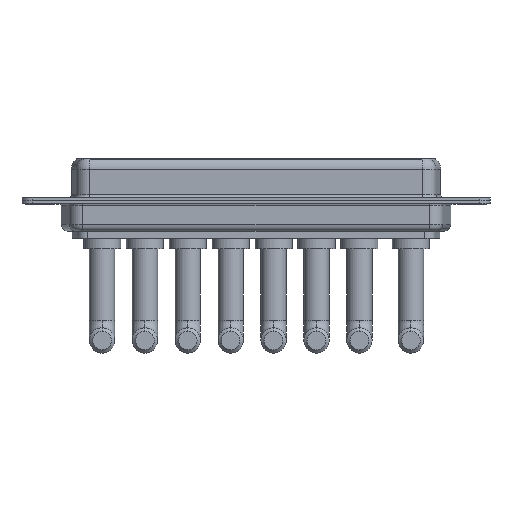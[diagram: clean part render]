
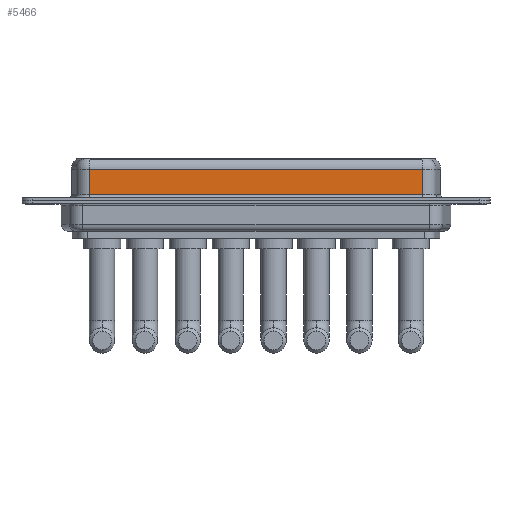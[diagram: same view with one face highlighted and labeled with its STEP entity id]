
A CAD part, front view. The second image highlights one B-rep face of the part: STEP entity #5466.
In plain terms, the highlighted planar face has unit normal (0, -1, 0).
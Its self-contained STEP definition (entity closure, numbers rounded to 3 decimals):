
#313 = ORIENTED_EDGE ( 'NONE', *, *, #11012, .F. ) ;
#325 = CARTESIAN_POINT ( 'NONE',  ( 7.038, -3.95, 0.9 ) ) ;
#837 = LINE ( 'NONE', #6211, #10198 ) ;
#909 = LINE ( 'NONE', #8097, #8647 ) ;
#1168 = EDGE_CURVE ( 'NONE', #10026, #2926, #10591, .T. ) ;
#1311 = ORIENTED_EDGE ( 'NONE', *, *, #1457, .T. ) ;
#1457 = EDGE_CURVE ( 'NONE', #5339, #10026, #9608, .T. ) ;
#2400 = CARTESIAN_POINT ( 'NONE',  ( 56.462, -3.95, 4.65 ) ) ;
#2618 = DIRECTION ( 'NONE',  ( 1., 0., 0. ) ) ;
#2660 = DIRECTION ( 'NONE',  ( 0., 0., -1. ) ) ;
#2926 = VERTEX_POINT ( 'NONE', #325 ) ;
#3051 = CARTESIAN_POINT ( 'NONE',  ( 56.462, -3.95, 6.4 ) ) ;
#3469 = ORIENTED_EDGE ( 'NONE', *, *, #6522, .T. ) ;
#4916 = DIRECTION ( 'NONE',  ( 0., 1., 0. ) ) ;
#4972 = DIRECTION ( 'NONE',  ( 0., 0., 1. ) ) ;
#5015 = CARTESIAN_POINT ( 'NONE',  ( 7.038, -3.95, 4.65 ) ) ;
#5339 = VERTEX_POINT ( 'NONE', #8720 ) ;
#5466 = ADVANCED_FACE ( 'NONE', ( #5605 ), #7546, .F. ) ;
#5553 = ORIENTED_EDGE ( 'NONE', *, *, #1168, .T. ) ;
#5587 = VECTOR ( 'NONE', #6182, 1000. ) ;
#5605 = FACE_OUTER_BOUND ( 'NONE', #8673, .T. ) ;
#5945 = CARTESIAN_POINT ( 'NONE',  ( 56.462, -3.95, 0.9 ) ) ;
#6182 = DIRECTION ( 'NONE',  ( 0., 0., -1. ) ) ;
#6211 = CARTESIAN_POINT ( 'NONE',  ( 56.462, -3.95, 6.4 ) ) ;
#6522 = EDGE_CURVE ( 'NONE', #2926, #10752, #909, .T. ) ;
#7086 = CARTESIAN_POINT ( 'NONE',  ( 7.038, -3.95, 6.4 ) ) ;
#7546 = PLANE ( 'NONE',  #10645 ) ;
#8097 = CARTESIAN_POINT ( 'NONE',  ( 56.462, -3.95, 0.9 ) ) ;
#8444 = VECTOR ( 'NONE', #11218, 1000. ) ;
#8647 = VECTOR ( 'NONE', #2618, 1000. ) ;
#8673 = EDGE_LOOP ( 'NONE', ( #313, #1311, #5553, #3469 ) ) ;
#8720 = CARTESIAN_POINT ( 'NONE',  ( 56.462, -3.95, 4.65 ) ) ;
#9608 = LINE ( 'NONE', #2400, #8444 ) ;
#10026 = VERTEX_POINT ( 'NONE', #5015 ) ;
#10198 = VECTOR ( 'NONE', #2660, 1000. ) ;
#10591 = LINE ( 'NONE', #7086, #5587 ) ;
#10645 = AXIS2_PLACEMENT_3D ( 'NONE', #3051, #4916, #4972 ) ;
#10752 = VERTEX_POINT ( 'NONE', #5945 ) ;
#11012 = EDGE_CURVE ( 'NONE', #5339, #10752, #837, .T. ) ;
#11218 = DIRECTION ( 'NONE',  ( -1., 0., 0. ) ) ;
